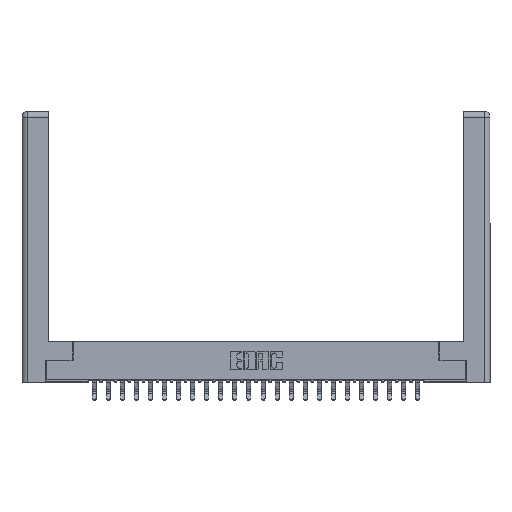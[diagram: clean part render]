
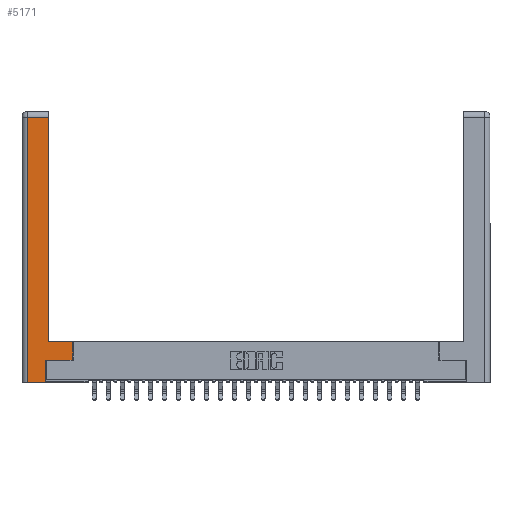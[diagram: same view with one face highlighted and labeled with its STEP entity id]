
A CAD part, top view. The second image highlights one B-rep face of the part: STEP entity #5171.
In plain terms, the highlighted planar face has unit normal (0, 0, 1).
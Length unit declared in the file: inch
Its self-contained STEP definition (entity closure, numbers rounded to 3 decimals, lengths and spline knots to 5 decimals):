
#233 = CARTESIAN_POINT ( 'NONE',  ( 0.265, 0., 0. ) ) ;
#251 = EDGE_CURVE ( 'NONE', #16911, #20301, #27652, .T. ) ;
#368 = VERTEX_POINT ( 'NONE', #20060 ) ;
#735 = LINE ( 'NONE', #233, #8948 ) ;
#1242 = EDGE_CURVE ( 'NONE', #20774, #368, #3698, .T. ) ;
#1477 = CARTESIAN_POINT ( 'NONE',  ( 0.295, 0.45, 0. ) ) ;
#2423 = LINE ( 'NONE', #15730, #27976 ) ;
#3089 = VECTOR ( 'NONE', #17886, 39.37008 ) ;
#3393 = CARTESIAN_POINT ( 'NONE',  ( 0.265, 0.245, 0. ) ) ;
#3476 = DIRECTION ( 'NONE',  ( 0., -1., 0. ) ) ;
#3698 = LINE ( 'NONE', #29237, #8979 ) ;
#4695 = CARTESIAN_POINT ( 'NONE',  ( 0.565, 0.45, 0. ) ) ;
#4882 = DIRECTION ( 'NONE',  ( 1., 0., 0. ) ) ;
#5171 = ADVANCED_FACE ( 'NONE', ( #30501 ), #27176, .F. ) ;
#5493 = EDGE_CURVE ( 'NONE', #368, #6221, #16589, .T. ) ;
#5515 = LINE ( 'NONE', #25862, #14859 ) ;
#5723 = CARTESIAN_POINT ( 'NONE',  ( 0.565, 0.45, 0. ) ) ;
#6046 = ORIENTED_EDGE ( 'NONE', *, *, #29309, .T. ) ;
#6118 = CARTESIAN_POINT ( 'NONE',  ( 0.295, 0.45, 0. ) ) ;
#6221 = VERTEX_POINT ( 'NONE', #4695 ) ;
#7418 = EDGE_CURVE ( 'NONE', #6221, #16911, #10470, .T. ) ;
#7763 = CARTESIAN_POINT ( 'NONE',  ( 0.0615, 2.94, 0. ) ) ;
#8388 = DIRECTION ( 'NONE',  ( 0., 0., -1. ) ) ;
#8437 = VERTEX_POINT ( 'NONE', #7763 ) ;
#8948 = VECTOR ( 'NONE', #4882, 39.37008 ) ;
#8979 = VECTOR ( 'NONE', #19343, 39.37008 ) ;
#10470 = LINE ( 'NONE', #6118, #16090 ) ;
#10520 = DIRECTION ( 'NONE',  ( 0., 1., 0. ) ) ;
#10541 = EDGE_CURVE ( 'NONE', #21422, #20774, #31005, .T. ) ;
#11114 = ORIENTED_EDGE ( 'NONE', *, *, #1242, .T. ) ;
#11905 = EDGE_LOOP ( 'NONE', ( #15440, #15646, #27381, #6046, #20959, #11114, #24325, #27012 ) ) ;
#12098 = CARTESIAN_POINT ( 'NONE',  ( 0.265, 0.245, 0. ) ) ;
#13712 = VECTOR ( 'NONE', #10520, 39.37008 ) ;
#14859 = VECTOR ( 'NONE', #18811, 39.37008 ) ;
#15384 = CARTESIAN_POINT ( 'NONE',  ( 0., 0., 0. ) ) ;
#15440 = ORIENTED_EDGE ( 'NONE', *, *, #251, .T. ) ;
#15646 = ORIENTED_EDGE ( 'NONE', *, *, #23451, .T. ) ;
#15730 = CARTESIAN_POINT ( 'NONE',  ( 0.0615, 0., 0. ) ) ;
#16090 = VECTOR ( 'NONE', #18057, 39.37008 ) ;
#16589 = LINE ( 'NONE', #5723, #3089 ) ;
#16911 = VERTEX_POINT ( 'NONE', #1477 ) ;
#17638 = CARTESIAN_POINT ( 'NONE',  ( 0.0615, 0., 0. ) ) ;
#17886 = DIRECTION ( 'NONE',  ( 0., 1., 0. ) ) ;
#18057 = DIRECTION ( 'NONE',  ( -1., 0., 0. ) ) ;
#18811 = DIRECTION ( 'NONE',  ( -1., 0., 0. ) ) ;
#19020 = EDGE_CURVE ( 'NONE', #8437, #25262, #2423, .T. ) ;
#19343 = DIRECTION ( 'NONE',  ( 1., 0., 0. ) ) ;
#19416 = CARTESIAN_POINT ( 'NONE',  ( 0.295, 3., 0. ) ) ;
#19729 = DIRECTION ( 'NONE',  ( 0., 1., 0. ) ) ;
#19903 = DIRECTION ( 'NONE',  ( -1., 0., 0. ) ) ;
#20060 = CARTESIAN_POINT ( 'NONE',  ( 0.565, 0.245, 0. ) ) ;
#20301 = VERTEX_POINT ( 'NONE', #27304 ) ;
#20774 = VERTEX_POINT ( 'NONE', #12098 ) ;
#20959 = ORIENTED_EDGE ( 'NONE', *, *, #10541, .T. ) ;
#21422 = VERTEX_POINT ( 'NONE', #22942 ) ;
#22942 = CARTESIAN_POINT ( 'NONE',  ( 0.265, 0., 0. ) ) ;
#23451 = EDGE_CURVE ( 'NONE', #20301, #8437, #5515, .T. ) ;
#24325 = ORIENTED_EDGE ( 'NONE', *, *, #5493, .T. ) ;
#25262 = VERTEX_POINT ( 'NONE', #17638 ) ;
#25862 = CARTESIAN_POINT ( 'NONE',  ( 0.0615, 2.94, 0. ) ) ;
#26844 = VECTOR ( 'NONE', #19729, 39.37008 ) ;
#27012 = ORIENTED_EDGE ( 'NONE', *, *, #7418, .T. ) ;
#27176 = PLANE ( 'NONE',  #29223 ) ;
#27304 = CARTESIAN_POINT ( 'NONE',  ( 0.295, 2.94, 0. ) ) ;
#27381 = ORIENTED_EDGE ( 'NONE', *, *, #19020, .T. ) ;
#27652 = LINE ( 'NONE', #19416, #26844 ) ;
#27976 = VECTOR ( 'NONE', #3476, 39.37008 ) ;
#29223 = AXIS2_PLACEMENT_3D ( 'NONE', #15384, #8388, #19903 ) ;
#29237 = CARTESIAN_POINT ( 'NONE',  ( 0.565, 0.245, 0. ) ) ;
#29309 = EDGE_CURVE ( 'NONE', #25262, #21422, #735, .T. ) ;
#30501 = FACE_OUTER_BOUND ( 'NONE', #11905, .T. ) ;
#31005 = LINE ( 'NONE', #3393, #13712 ) ;
